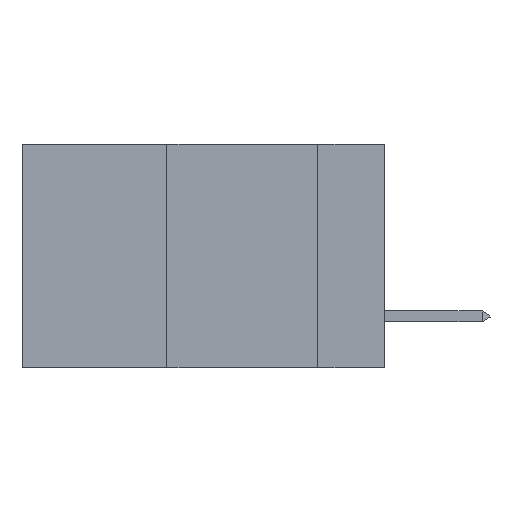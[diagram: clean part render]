
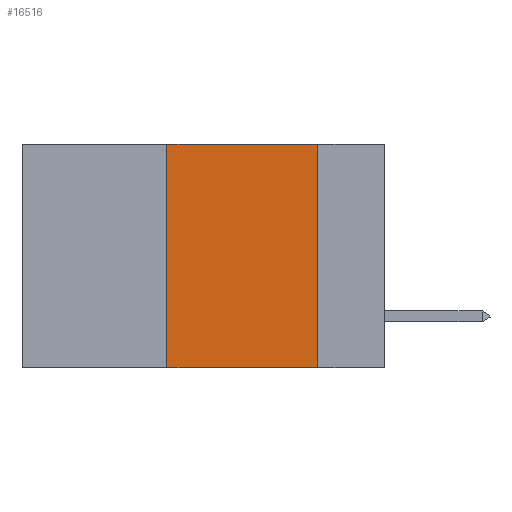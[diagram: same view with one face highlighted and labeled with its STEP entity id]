
A CAD part, left-side view. The second image highlights one B-rep face of the part: STEP entity #16516.
In plain terms, the highlighted planar face has unit normal (-1, 0, 0).
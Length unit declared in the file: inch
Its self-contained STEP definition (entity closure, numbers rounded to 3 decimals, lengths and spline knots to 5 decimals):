
#344 = DIRECTION ( 'NONE',  ( 0., -1., 0. ) ) ;
#678 = CARTESIAN_POINT ( 'NONE',  ( 0., 0.6, 0. ) ) ;
#2127 = CARTESIAN_POINT ( 'NONE',  ( 0., 0.6, -0.37 ) ) ;
#4169 = VERTEX_POINT ( 'NONE', #24815 ) ;
#4469 = VERTEX_POINT ( 'NONE', #28351 ) ;
#6697 = LINE ( 'NONE', #24456, #31110 ) ;
#7143 = EDGE_CURVE ( 'NONE', #16340, #10788, #18159, .T. ) ;
#7286 = CARTESIAN_POINT ( 'NONE',  ( 0., 0.11, 0. ) ) ;
#9448 = ORIENTED_EDGE ( 'NONE', *, *, #28157, .T. ) ;
#9616 = EDGE_CURVE ( 'NONE', #10788, #4469, #18580, .T. ) ;
#10788 = VERTEX_POINT ( 'NONE', #7286 ) ;
#11878 = CARTESIAN_POINT ( 'NONE',  ( 0., 0.6, 0. ) ) ;
#15573 = EDGE_LOOP ( 'NONE', ( #34339, #33140, #26727, #9448 ) ) ;
#15939 = CARTESIAN_POINT ( 'NONE',  ( 0., 0.11, 0. ) ) ;
#16340 = VERTEX_POINT ( 'NONE', #37823 ) ;
#16516 = ADVANCED_FACE ( 'NONE', ( #27127 ), #32721, .F. ) ;
#17967 = DIRECTION ( 'NONE',  ( 1., 0., 0. ) ) ;
#18159 = LINE ( 'NONE', #678, #23823 ) ;
#18580 = LINE ( 'NONE', #15939, #36453 ) ;
#18949 = EDGE_CURVE ( 'NONE', #4169, #16340, #6697, .T. ) ;
#20609 = VECTOR ( 'NONE', #28505, 39.37008 ) ;
#23823 = VECTOR ( 'NONE', #344, 39.37008 ) ;
#24456 = CARTESIAN_POINT ( 'NONE',  ( 0., 0.36, 0. ) ) ;
#24689 = DIRECTION ( 'NONE',  ( 0., 0., -1. ) ) ;
#24815 = CARTESIAN_POINT ( 'NONE',  ( 0., 0.36, -0.37 ) ) ;
#26022 = AXIS2_PLACEMENT_3D ( 'NONE', #11878, #17967, #26959 ) ;
#26727 = ORIENTED_EDGE ( 'NONE', *, *, #18949, .F. ) ;
#26959 = DIRECTION ( 'NONE',  ( 0., 0., -1. ) ) ;
#27127 = FACE_OUTER_BOUND ( 'NONE', #15573, .T. ) ;
#28157 = EDGE_CURVE ( 'NONE', #4169, #4469, #34364, .T. ) ;
#28351 = CARTESIAN_POINT ( 'NONE',  ( 0., 0.11, -0.37 ) ) ;
#28505 = DIRECTION ( 'NONE',  ( 0., -1., 0. ) ) ;
#31110 = VECTOR ( 'NONE', #32898, 39.37008 ) ;
#32721 = PLANE ( 'NONE',  #26022 ) ;
#32898 = DIRECTION ( 'NONE',  ( 0., 0., 1. ) ) ;
#33140 = ORIENTED_EDGE ( 'NONE', *, *, #7143, .F. ) ;
#34339 = ORIENTED_EDGE ( 'NONE', *, *, #9616, .F. ) ;
#34364 = LINE ( 'NONE', #2127, #20609 ) ;
#36453 = VECTOR ( 'NONE', #24689, 39.37008 ) ;
#37823 = CARTESIAN_POINT ( 'NONE',  ( 0., 0.36, 0. ) ) ;
